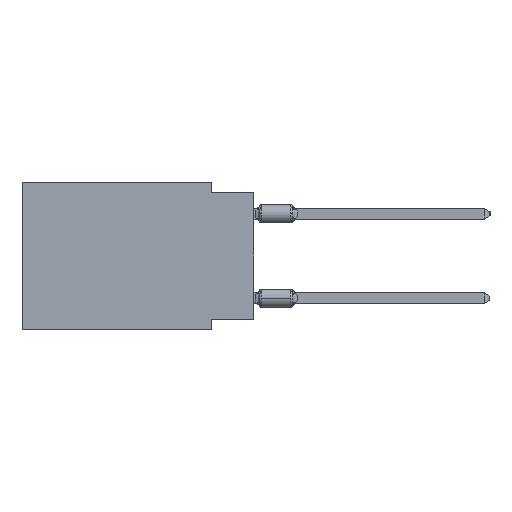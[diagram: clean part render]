
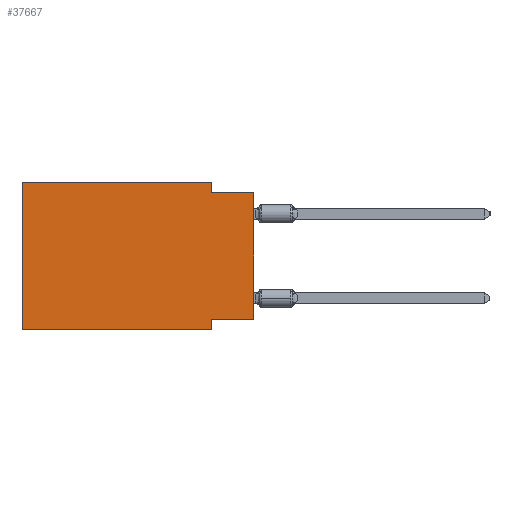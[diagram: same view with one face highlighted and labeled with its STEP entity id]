
A CAD part, left-side view. The second image highlights one B-rep face of the part: STEP entity #37667.
In plain terms, the highlighted planar face has unit normal (-1, 0, 0).
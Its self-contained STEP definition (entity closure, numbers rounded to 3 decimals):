
#6633 = ORIENTED_EDGE ( 'NONE', *, *, #51207, .F. ) ;
#7837 = LINE ( 'NONE', #23424, #52593 ) ;
#8251 = ORIENTED_EDGE ( 'NONE', *, *, #41704, .F. ) ;
#9256 = LINE ( 'NONE', #37619, #13989 ) ;
#11010 = EDGE_CURVE ( 'NONE', #58766, #28859, #30648, .T. ) ;
#11189 = ORIENTED_EDGE ( 'NONE', *, *, #27478, .F. ) ;
#11603 = VECTOR ( 'NONE', #46331, 1000. ) ;
#12408 = CARTESIAN_POINT ( 'NONE',  ( 0., 2.54, 0. ) ) ;
#13732 = CARTESIAN_POINT ( 'NONE',  ( 0., 2.54, 0. ) ) ;
#13989 = VECTOR ( 'NONE', #62149, 1000. ) ;
#16312 = CARTESIAN_POINT ( 'NONE',  ( 0., 2.54, -8.89 ) ) ;
#16460 = EDGE_CURVE ( 'NONE', #33229, #53461, #40607, .T. ) ;
#16935 = DIRECTION ( 'NONE',  ( 0., 0., -1. ) ) ;
#18720 = LINE ( 'NONE', #61119, #61828 ) ;
#18890 = ORIENTED_EDGE ( 'NONE', *, *, #43524, .T. ) ;
#19086 = FACE_OUTER_BOUND ( 'NONE', #31486, .T. ) ;
#19740 = VERTEX_POINT ( 'NONE', #56744 ) ;
#23239 = DIRECTION ( 'NONE',  ( 1., 0., 0. ) ) ;
#23339 = CARTESIAN_POINT ( 'NONE',  ( 0., 2.54, -8.255 ) ) ;
#23424 = CARTESIAN_POINT ( 'NONE',  ( 0., 0., -0.635 ) ) ;
#24267 = LINE ( 'NONE', #27809, #41542 ) ;
#25050 = VECTOR ( 'NONE', #16935, 1000. ) ;
#25502 = ORIENTED_EDGE ( 'NONE', *, *, #48709, .F. ) ;
#26504 = ORIENTED_EDGE ( 'NONE', *, *, #43079, .F. ) ;
#27043 = DIRECTION ( 'NONE',  ( 0., 0., -1. ) ) ;
#27478 = EDGE_CURVE ( 'NONE', #32149, #61784, #9256, .T. ) ;
#27689 = LINE ( 'NONE', #12408, #47724 ) ;
#27809 = CARTESIAN_POINT ( 'NONE',  ( 0., 13.97, -8.89 ) ) ;
#28859 = VERTEX_POINT ( 'NONE', #47532 ) ;
#29810 = LINE ( 'NONE', #54637, #32222 ) ;
#30648 = LINE ( 'NONE', #16312, #25050 ) ;
#31486 = EDGE_LOOP ( 'NONE', ( #61811, #25502, #6633, #11189, #26504, #18890, #58177, #8251 ) ) ;
#32149 = VERTEX_POINT ( 'NONE', #56132 ) ;
#32222 = VECTOR ( 'NONE', #43846, 1000. ) ;
#32753 = DIRECTION ( 'NONE',  ( 0., 0., 1. ) ) ;
#33229 = VERTEX_POINT ( 'NONE', #43787 ) ;
#37619 = CARTESIAN_POINT ( 'NONE',  ( 0., 13.97, 0. ) ) ;
#37667 = ADVANCED_FACE ( 'NONE', ( #19086 ), #57639, .F. ) ;
#37768 = DIRECTION ( 'NONE',  ( 0., -1., 0. ) ) ;
#38511 = DIRECTION ( 'NONE',  ( 0., 0., -1. ) ) ;
#39848 = CARTESIAN_POINT ( 'NONE',  ( 0., 13.97, -8.89 ) ) ;
#40607 = LINE ( 'NONE', #45698, #11603 ) ;
#41542 = VECTOR ( 'NONE', #48168, 1000. ) ;
#41704 = EDGE_CURVE ( 'NONE', #33229, #58766, #29810, .T. ) ;
#43079 = EDGE_CURVE ( 'NONE', #55094, #32149, #18720, .T. ) ;
#43524 = EDGE_CURVE ( 'NONE', #55094, #28859, #24267, .T. ) ;
#43787 = CARTESIAN_POINT ( 'NONE',  ( 0., 0., -8.255 ) ) ;
#43846 = DIRECTION ( 'NONE',  ( 0., 1., 0. ) ) ;
#45698 = CARTESIAN_POINT ( 'NONE',  ( 0., 0., 0. ) ) ;
#46331 = DIRECTION ( 'NONE',  ( 0., 0., 1. ) ) ;
#47532 = CARTESIAN_POINT ( 'NONE',  ( 0., 2.54, -8.89 ) ) ;
#47724 = VECTOR ( 'NONE', #27043, 1000. ) ;
#48168 = DIRECTION ( 'NONE',  ( 0., -1., 0. ) ) ;
#48709 = EDGE_CURVE ( 'NONE', #19740, #53461, #7837, .T. ) ;
#51207 = EDGE_CURVE ( 'NONE', #61784, #19740, #27689, .T. ) ;
#52593 = VECTOR ( 'NONE', #37768, 1000. ) ;
#53461 = VERTEX_POINT ( 'NONE', #58100 ) ;
#54637 = CARTESIAN_POINT ( 'NONE',  ( 0., 0., -8.255 ) ) ;
#55094 = VERTEX_POINT ( 'NONE', #39848 ) ;
#56132 = CARTESIAN_POINT ( 'NONE',  ( 0., 13.97, 0. ) ) ;
#56239 = AXIS2_PLACEMENT_3D ( 'NONE', #62421, #23239, #38511 ) ;
#56744 = CARTESIAN_POINT ( 'NONE',  ( 0., 2.54, -0.635 ) ) ;
#57639 = PLANE ( 'NONE',  #56239 ) ;
#58100 = CARTESIAN_POINT ( 'NONE',  ( 0., 0., -0.635 ) ) ;
#58177 = ORIENTED_EDGE ( 'NONE', *, *, #11010, .F. ) ;
#58766 = VERTEX_POINT ( 'NONE', #23339 ) ;
#61119 = CARTESIAN_POINT ( 'NONE',  ( 0., 13.97, 0. ) ) ;
#61784 = VERTEX_POINT ( 'NONE', #13732 ) ;
#61811 = ORIENTED_EDGE ( 'NONE', *, *, #16460, .T. ) ;
#61828 = VECTOR ( 'NONE', #32753, 1000. ) ;
#62149 = DIRECTION ( 'NONE',  ( 0., -1., 0. ) ) ;
#62421 = CARTESIAN_POINT ( 'NONE',  ( 0., 13.97, 0. ) ) ;
